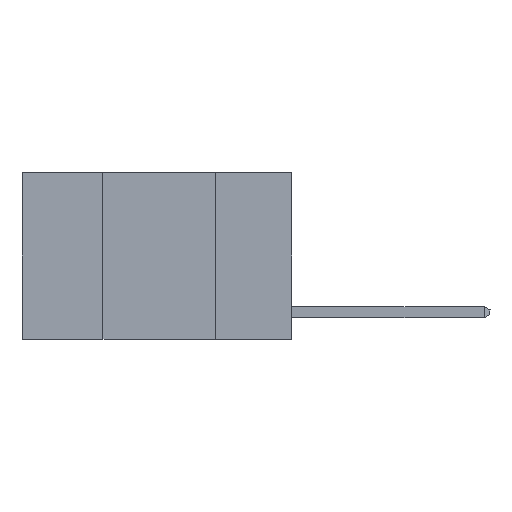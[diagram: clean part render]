
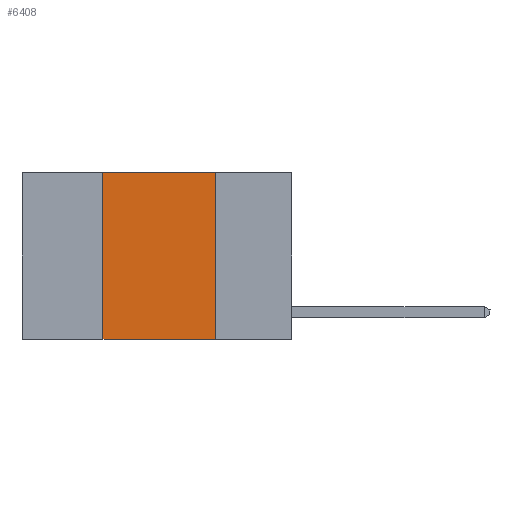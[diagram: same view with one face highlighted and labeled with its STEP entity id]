
A CAD part, left-side view. The second image highlights one B-rep face of the part: STEP entity #6408.
In plain terms, the highlighted planar face has unit normal (-1, 0, 0).
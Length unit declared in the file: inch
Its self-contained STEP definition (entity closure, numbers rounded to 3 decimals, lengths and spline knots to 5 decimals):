
#222 = CARTESIAN_POINT ( 'NONE',  ( 0., 0.17, 0. ) ) ;
#331 = DIRECTION ( 'NONE',  ( 0., -1., 0. ) ) ;
#376 = EDGE_CURVE ( 'NONE', #1239, #6255, #3083, .T. ) ;
#1117 = ORIENTED_EDGE ( 'NONE', *, *, #3670, .F. ) ;
#1178 = CARTESIAN_POINT ( 'NONE',  ( 0., 0.17, 0. ) ) ;
#1239 = VERTEX_POINT ( 'NONE', #1383 ) ;
#1383 = CARTESIAN_POINT ( 'NONE',  ( 0., 0.42, -0.37 ) ) ;
#1406 = CARTESIAN_POINT ( 'NONE',  ( 0., 0.6, 0. ) ) ;
#2484 = EDGE_CURVE ( 'NONE', #7083, #3325, #12149, .T. ) ;
#2992 = VECTOR ( 'NONE', #8929, 39.37008 ) ;
#3083 = LINE ( 'NONE', #4186, #9950 ) ;
#3109 = DIRECTION ( 'NONE',  ( 1., 0., 0. ) ) ;
#3325 = VERTEX_POINT ( 'NONE', #6771 ) ;
#3557 = CARTESIAN_POINT ( 'NONE',  ( 0., 0.42, 0. ) ) ;
#3670 = EDGE_CURVE ( 'NONE', #6255, #7083, #10419, .T. ) ;
#3948 = PLANE ( 'NONE',  #5542 ) ;
#4186 = CARTESIAN_POINT ( 'NONE',  ( 0., 0.42, 0. ) ) ;
#4586 = ORIENTED_EDGE ( 'NONE', *, *, #376, .F. ) ;
#5542 = AXIS2_PLACEMENT_3D ( 'NONE', #6117, #3109, #9341 ) ;
#6117 = CARTESIAN_POINT ( 'NONE',  ( 0., 0.6, 0. ) ) ;
#6221 = DIRECTION ( 'NONE',  ( 0., 0., 1. ) ) ;
#6255 = VERTEX_POINT ( 'NONE', #3557 ) ;
#6408 = ADVANCED_FACE ( 'NONE', ( #8243 ), #3948, .F. ) ;
#6490 = EDGE_CURVE ( 'NONE', #1239, #3325, #10175, .T. ) ;
#6771 = CARTESIAN_POINT ( 'NONE',  ( 0., 0.17, -0.37 ) ) ;
#7083 = VERTEX_POINT ( 'NONE', #222 ) ;
#7355 = VECTOR ( 'NONE', #331, 39.37008 ) ;
#7366 = EDGE_LOOP ( 'NONE', ( #9412, #1117, #4586, #12964 ) ) ;
#7854 = CARTESIAN_POINT ( 'NONE',  ( 0., 0.6, -0.37 ) ) ;
#8243 = FACE_OUTER_BOUND ( 'NONE', #7366, .T. ) ;
#8929 = DIRECTION ( 'NONE',  ( 0., -1., 0. ) ) ;
#9341 = DIRECTION ( 'NONE',  ( 0., 0., -1. ) ) ;
#9412 = ORIENTED_EDGE ( 'NONE', *, *, #2484, .F. ) ;
#9474 = VECTOR ( 'NONE', #11357, 39.37008 ) ;
#9950 = VECTOR ( 'NONE', #6221, 39.37008 ) ;
#10175 = LINE ( 'NONE', #7854, #2992 ) ;
#10419 = LINE ( 'NONE', #1406, #7355 ) ;
#11357 = DIRECTION ( 'NONE',  ( 0., 0., -1. ) ) ;
#12149 = LINE ( 'NONE', #1178, #9474 ) ;
#12964 = ORIENTED_EDGE ( 'NONE', *, *, #6490, .T. ) ;
